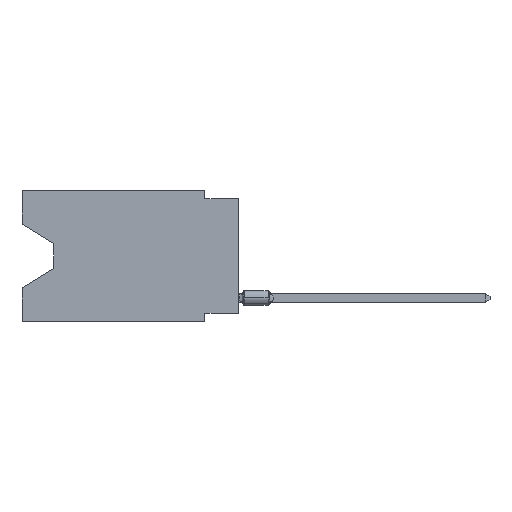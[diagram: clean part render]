
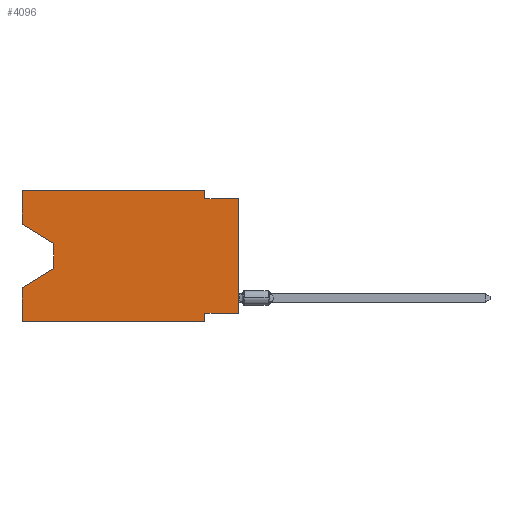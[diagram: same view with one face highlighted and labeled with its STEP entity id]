
A CAD part, left-side view. The second image highlights one B-rep face of the part: STEP entity #4096.
In plain terms, the highlighted planar face has unit normal (-1, 0, 0).
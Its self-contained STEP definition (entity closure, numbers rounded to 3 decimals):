
#194 = LINE ( 'NONE', #21849, #23102 ) ;
#578 = ORIENTED_EDGE ( 'NONE', *, *, #12526, .F. ) ;
#713 = CARTESIAN_POINT ( 'NONE',  ( 0., 0., -0.635 ) ) ;
#933 = FACE_OUTER_BOUND ( 'NONE', #3299, .T. ) ;
#1476 = LINE ( 'NONE', #23614, #26637 ) ;
#2324 = DIRECTION ( 'NONE',  ( 0., 0., -1. ) ) ;
#2398 = VECTOR ( 'NONE', #2324, 1000. ) ;
#3292 = ORIENTED_EDGE ( 'NONE', *, *, #23097, .F. ) ;
#3299 = EDGE_LOOP ( 'NONE', ( #27702, #21136, #19766, #578, #30847, #30477, #19969, #28740, #23885, #3292, #26623, #31809 ) ) ;
#3979 = LINE ( 'NONE', #30514, #24448 ) ;
#4096 = ADVANCED_FACE ( 'NONE', ( #933 ), #5937, .F. ) ;
#4141 = DIRECTION ( 'NONE',  ( 0., -1., 0. ) ) ;
#4201 = DIRECTION ( 'NONE',  ( 0., 0., -1. ) ) ;
#4330 = VECTOR ( 'NONE', #22580, 1000. ) ;
#4570 = CARTESIAN_POINT ( 'NONE',  ( 0., 2.54, 0. ) ) ;
#5286 = LINE ( 'NONE', #15151, #4330 ) ;
#5641 = DIRECTION ( 'NONE',  ( 0., -0.855, -0.519 ) ) ;
#5757 = DIRECTION ( 'NONE',  ( 0., 1., 0. ) ) ;
#5937 = PLANE ( 'NONE',  #23787 ) ;
#7288 = EDGE_CURVE ( 'NONE', #28272, #17023, #9521, .T. ) ;
#7299 = DIRECTION ( 'NONE',  ( 0., 0., 1. ) ) ;
#8689 = CARTESIAN_POINT ( 'NONE',  ( 0., 16.383, 0. ) ) ;
#9521 = LINE ( 'NONE', #28942, #29442 ) ;
#9739 = VERTEX_POINT ( 'NONE', #27280 ) ;
#9903 = LINE ( 'NONE', #4570, #2398 ) ;
#10933 = DIRECTION ( 'NONE',  ( 0., 0., -1. ) ) ;
#11252 = DIRECTION ( 'NONE',  ( 1., 0., 0. ) ) ;
#11567 = DIRECTION ( 'NONE',  ( 0., 0., -1. ) ) ;
#11624 = VECTOR ( 'NONE', #11567, 1000. ) ;
#11641 = LINE ( 'NONE', #19078, #17647 ) ;
#11861 = LINE ( 'NONE', #16891, #11624 ) ;
#12522 = EDGE_CURVE ( 'NONE', #9739, #13287, #23759, .T. ) ;
#12526 = EDGE_CURVE ( 'NONE', #13656, #27904, #11641, .T. ) ;
#12876 = CARTESIAN_POINT ( 'NONE',  ( 0., 13.97, -5.893 ) ) ;
#13287 = VERTEX_POINT ( 'NONE', #16534 ) ;
#13296 = VERTEX_POINT ( 'NONE', #26567 ) ;
#13355 = DIRECTION ( 'NONE',  ( 0., 0.855, -0.519 ) ) ;
#13518 = VECTOR ( 'NONE', #4201, 1000. ) ;
#13656 = VERTEX_POINT ( 'NONE', #14534 ) ;
#13846 = LINE ( 'NONE', #21130, #19937 ) ;
#14026 = EDGE_CURVE ( 'NONE', #22085, #25926, #27817, .T. ) ;
#14534 = CARTESIAN_POINT ( 'NONE',  ( 0., 16.383, -9.906 ) ) ;
#14861 = VECTOR ( 'NONE', #5641, 1000. ) ;
#14890 = CARTESIAN_POINT ( 'NONE',  ( 0., 13.97, -4.013 ) ) ;
#15151 = CARTESIAN_POINT ( 'NONE',  ( 0., 16.383, 0. ) ) ;
#16490 = CARTESIAN_POINT ( 'NONE',  ( 0., 2.54, -9.906 ) ) ;
#16534 = CARTESIAN_POINT ( 'NONE',  ( 0., 2.54, -9.906 ) ) ;
#16631 = EDGE_CURVE ( 'NONE', #25075, #27904, #30023, .T. ) ;
#16891 = CARTESIAN_POINT ( 'NONE',  ( 0., 13.97, -4.013 ) ) ;
#17023 = VERTEX_POINT ( 'NONE', #713 ) ;
#17647 = VECTOR ( 'NONE', #31532, 1000. ) ;
#17962 = VERTEX_POINT ( 'NONE', #8689 ) ;
#19052 = CARTESIAN_POINT ( 'NONE',  ( 0., 2.54, -0.635 ) ) ;
#19078 = CARTESIAN_POINT ( 'NONE',  ( 0., 16.383, 0. ) ) ;
#19388 = CARTESIAN_POINT ( 'NONE',  ( 0., 13.97, -5.893 ) ) ;
#19419 = EDGE_CURVE ( 'NONE', #22085, #17962, #5286, .T. ) ;
#19446 = EDGE_CURVE ( 'NONE', #13296, #9739, #3979, .T. ) ;
#19648 = EDGE_CURVE ( 'NONE', #25926, #25075, #11861, .T. ) ;
#19766 = ORIENTED_EDGE ( 'NONE', *, *, #16631, .T. ) ;
#19937 = VECTOR ( 'NONE', #4141, 1000. ) ;
#19969 = ORIENTED_EDGE ( 'NONE', *, *, #19446, .F. ) ;
#20114 = VERTEX_POINT ( 'NONE', #26875 ) ;
#20379 = EDGE_CURVE ( 'NONE', #13656, #13287, #1476, .T. ) ;
#21130 = CARTESIAN_POINT ( 'NONE',  ( 0., 16.383, 0. ) ) ;
#21136 = ORIENTED_EDGE ( 'NONE', *, *, #19648, .T. ) ;
#21785 = CARTESIAN_POINT ( 'NONE',  ( 0., 16.383, -2.546 ) ) ;
#21849 = CARTESIAN_POINT ( 'NONE',  ( 0., 0., 0. ) ) ;
#22085 = VERTEX_POINT ( 'NONE', #21785 ) ;
#22580 = DIRECTION ( 'NONE',  ( 0., 0., 1. ) ) ;
#22778 = EDGE_CURVE ( 'NONE', #13296, #17023, #194, .T. ) ;
#23097 = EDGE_CURVE ( 'NONE', #20114, #28272, #9903, .T. ) ;
#23102 = VECTOR ( 'NONE', #7299, 1000. ) ;
#23614 = CARTESIAN_POINT ( 'NONE',  ( 0., 16.383, -9.906 ) ) ;
#23759 = LINE ( 'NONE', #16490, #13518 ) ;
#23787 = AXIS2_PLACEMENT_3D ( 'NONE', #30686, #11252, #10933 ) ;
#23885 = ORIENTED_EDGE ( 'NONE', *, *, #7288, .F. ) ;
#24448 = VECTOR ( 'NONE', #5757, 1000. ) ;
#25075 = VERTEX_POINT ( 'NONE', #19388 ) ;
#25926 = VERTEX_POINT ( 'NONE', #14890 ) ;
#26207 = DIRECTION ( 'NONE',  ( 0., -1., 0. ) ) ;
#26567 = CARTESIAN_POINT ( 'NONE',  ( 0., 0., -9.271 ) ) ;
#26623 = ORIENTED_EDGE ( 'NONE', *, *, #28658, .F. ) ;
#26637 = VECTOR ( 'NONE', #26207, 1000. ) ;
#26875 = CARTESIAN_POINT ( 'NONE',  ( 0., 2.54, 0. ) ) ;
#27173 = DIRECTION ( 'NONE',  ( 0., -1., 0. ) ) ;
#27280 = CARTESIAN_POINT ( 'NONE',  ( 0., 2.54, -9.271 ) ) ;
#27702 = ORIENTED_EDGE ( 'NONE', *, *, #14026, .T. ) ;
#27817 = LINE ( 'NONE', #28293, #14861 ) ;
#27904 = VERTEX_POINT ( 'NONE', #28490 ) ;
#28272 = VERTEX_POINT ( 'NONE', #19052 ) ;
#28293 = CARTESIAN_POINT ( 'NONE',  ( 0., 16.383, -2.546 ) ) ;
#28490 = CARTESIAN_POINT ( 'NONE',  ( 0., 16.383, -7.36 ) ) ;
#28658 = EDGE_CURVE ( 'NONE', #17962, #20114, #13846, .T. ) ;
#28740 = ORIENTED_EDGE ( 'NONE', *, *, #22778, .T. ) ;
#28942 = CARTESIAN_POINT ( 'NONE',  ( 0., 0., -0.635 ) ) ;
#29442 = VECTOR ( 'NONE', #27173, 1000. ) ;
#30023 = LINE ( 'NONE', #12876, #31217 ) ;
#30477 = ORIENTED_EDGE ( 'NONE', *, *, #12522, .F. ) ;
#30514 = CARTESIAN_POINT ( 'NONE',  ( 0., 0., -9.271 ) ) ;
#30686 = CARTESIAN_POINT ( 'NONE',  ( 0., 16.383, 0. ) ) ;
#30847 = ORIENTED_EDGE ( 'NONE', *, *, #20379, .T. ) ;
#31217 = VECTOR ( 'NONE', #13355, 1000. ) ;
#31532 = DIRECTION ( 'NONE',  ( 0., 0., 1. ) ) ;
#31809 = ORIENTED_EDGE ( 'NONE', *, *, #19419, .F. ) ;
